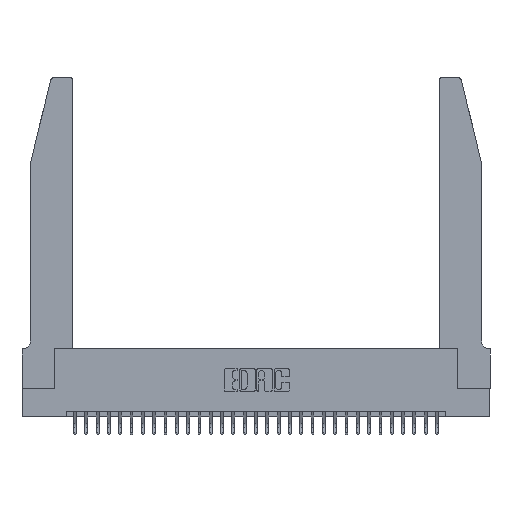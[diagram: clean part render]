
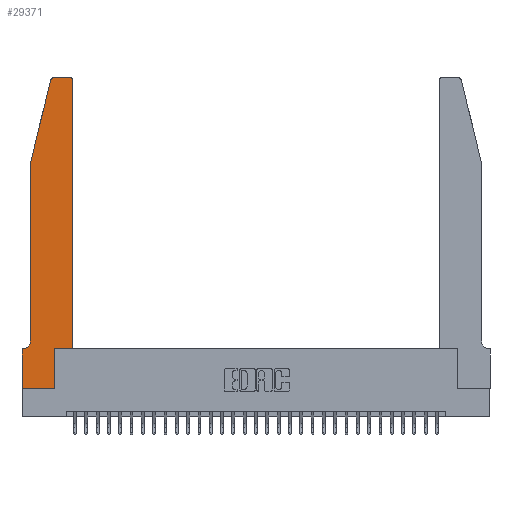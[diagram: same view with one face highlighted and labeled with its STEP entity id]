
A CAD part, top view. The second image highlights one B-rep face of the part: STEP entity #29371.
In plain terms, the highlighted planar face has unit normal (0, 0, 1).
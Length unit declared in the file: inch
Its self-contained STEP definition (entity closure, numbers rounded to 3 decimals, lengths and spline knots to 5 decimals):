
#147 = AXIS2_PLACEMENT_3D ( 'NONE', #3339, #28651, #21407 ) ;
#237 = ORIENTED_EDGE ( 'NONE', *, *, #23715, .T. ) ;
#705 = VERTEX_POINT ( 'NONE', #23378 ) ;
#1278 = VERTEX_POINT ( 'NONE', #14502 ) ;
#1462 = EDGE_CURVE ( 'NONE', #21361, #1278, #31575, .T. ) ;
#1588 = DIRECTION ( 'NONE',  ( -1., 0., 0. ) ) ;
#1649 = DIRECTION ( 'NONE',  ( -1., 0., 0. ) ) ;
#1764 = FACE_OUTER_BOUND ( 'NONE', #12556, .T. ) ;
#1934 = EDGE_CURVE ( 'NONE', #3386, #21623, #21065, .T. ) ;
#2164 = ORIENTED_EDGE ( 'NONE', *, *, #7362, .T. ) ;
#2233 = VERTEX_POINT ( 'NONE', #9811 ) ;
#2481 = CARTESIAN_POINT ( 'NONE',  ( 0., 0., 0.37 ) ) ;
#3025 = CIRCLE ( 'NONE', #10329, 0.07 ) ;
#3180 = ORIENTED_EDGE ( 'NONE', *, *, #1462, .T. ) ;
#3339 = CARTESIAN_POINT ( 'NONE',  ( 0.4205, 2.72, 0.37 ) ) ;
#3386 = VERTEX_POINT ( 'NONE', #26646 ) ;
#3661 = DIRECTION ( 'NONE',  ( 0., -1., 0. ) ) ;
#3945 = ORIENTED_EDGE ( 'NONE', *, *, #8197, .T. ) ;
#4258 = CARTESIAN_POINT ( 'NONE',  ( 0.284, 2.72, 0.37 ) ) ;
#4350 = CARTESIAN_POINT ( 'NONE',  ( 0., 0.35, 0.37 ) ) ;
#4453 = LINE ( 'NONE', #6448, #10668 ) ;
#4527 = CARTESIAN_POINT ( 'NONE',  ( 0., 0., 0.37 ) ) ;
#4607 = CARTESIAN_POINT ( 'NONE',  ( 0., 0.35, 0.37 ) ) ;
#4752 = DIRECTION ( 'NONE',  ( 0., -1., 0. ) ) ;
#5049 = AXIS2_PLACEMENT_3D ( 'NONE', #4258, #14022, #14249 ) ;
#5415 = ORIENTED_EDGE ( 'NONE', *, *, #1934, .T. ) ;
#5787 = CIRCLE ( 'NONE', #5049, 0.03 ) ;
#5803 = ORIENTED_EDGE ( 'NONE', *, *, #11107, .T. ) ;
#6448 = CARTESIAN_POINT ( 'NONE',  ( 0.0755, 0.35, 0.37 ) ) ;
#6578 = VERTEX_POINT ( 'NONE', #4350 ) ;
#6748 = DIRECTION ( 'NONE',  ( 1., 0., 0. ) ) ;
#6808 = ORIENTED_EDGE ( 'NONE', *, *, #9315, .T. ) ;
#6871 = DIRECTION ( 'NONE',  ( 0., 1., 0. ) ) ;
#6883 = LINE ( 'NONE', #14380, #18516 ) ;
#6910 = CARTESIAN_POINT ( 'NONE',  ( 0.2605, 2.75, 0.37 ) ) ;
#6927 = ORIENTED_EDGE ( 'NONE', *, *, #23131, .T. ) ;
#7362 = EDGE_CURVE ( 'NONE', #1278, #29435, #21138, .T. ) ;
#8197 = EDGE_CURVE ( 'NONE', #30524, #21361, #5787, .T. ) ;
#8481 = CARTESIAN_POINT ( 'NONE',  ( 0.4205, 2.75, 0.37 ) ) ;
#8822 = EDGE_CURVE ( 'NONE', #11421, #30524, #29008, .T. ) ;
#9034 = CARTESIAN_POINT ( 'NONE',  ( 0.2865, 0.35, 0.37 ) ) ;
#9295 = VECTOR ( 'NONE', #27070, 39.37008 ) ;
#9315 = EDGE_CURVE ( 'NONE', #705, #11421, #12741, .T. ) ;
#9405 = ORIENTED_EDGE ( 'NONE', *, *, #22620, .T. ) ;
#9459 = DIRECTION ( 'NONE',  ( 0., 0., 1. ) ) ;
#9489 = EDGE_CURVE ( 'NONE', #21623, #705, #6883, .T. ) ;
#9811 = CARTESIAN_POINT ( 'NONE',  ( 0.0055, 0.35, 0.37 ) ) ;
#10329 = AXIS2_PLACEMENT_3D ( 'NONE', #23628, #31355, #1649 ) ;
#10386 = ORIENTED_EDGE ( 'NONE', *, *, #28845, .T. ) ;
#10668 = VECTOR ( 'NONE', #1588, 39.37008 ) ;
#10918 = CARTESIAN_POINT ( 'NONE',  ( 0.0755, 2., 0.37 ) ) ;
#11107 = EDGE_CURVE ( 'NONE', #2233, #6578, #4453, .T. ) ;
#11223 = VECTOR ( 'NONE', #14382, 39.37008 ) ;
#11421 = VERTEX_POINT ( 'NONE', #8481 ) ;
#12450 = LINE ( 'NONE', #17221, #9295 ) ;
#12503 = AXIS2_PLACEMENT_3D ( 'NONE', #4607, #9459, #6748 ) ;
#12556 = EDGE_LOOP ( 'NONE', ( #21592, #3945, #3180, #2164, #237, #5803, #10386, #9405, #6927, #5415, #12750, #6808 ) ) ;
#12741 = CIRCLE ( 'NONE', #147, 0.03 ) ;
#12750 = ORIENTED_EDGE ( 'NONE', *, *, #9489, .T. ) ;
#14022 = DIRECTION ( 'NONE',  ( 0., 0., 1. ) ) ;
#14249 = DIRECTION ( 'NONE',  ( 1., 0., 0. ) ) ;
#14373 = PLANE ( 'NONE',  #12503 ) ;
#14380 = CARTESIAN_POINT ( 'NONE',  ( 0.4505, 0.35, 0.37 ) ) ;
#14382 = DIRECTION ( 'NONE',  ( 0., 1., 0. ) ) ;
#14502 = CARTESIAN_POINT ( 'NONE',  ( 0.0755, 2., 0.37 ) ) ;
#14812 = CARTESIAN_POINT ( 'NONE',  ( 0.0755, 0.42, 0.37 ) ) ;
#16044 = VECTOR ( 'NONE', #21302, 39.37008 ) ;
#16528 = VECTOR ( 'NONE', #4752, 39.37008 ) ;
#16774 = CARTESIAN_POINT ( 'NONE',  ( 0.25487, 2.72718, 0.37 ) ) ;
#17221 = CARTESIAN_POINT ( 'NONE',  ( 0., 0., 0.37 ) ) ;
#18432 = VECTOR ( 'NONE', #3661, 39.37008 ) ;
#18516 = VECTOR ( 'NONE', #6871, 39.37008 ) ;
#18690 = CARTESIAN_POINT ( 'NONE',  ( 0.0755, 2., 0.37 ) ) ;
#19278 = DIRECTION ( 'NONE',  ( -1., 0., 0. ) ) ;
#20878 = CARTESIAN_POINT ( 'NONE',  ( 0.4505, 0.35, 0.37 ) ) ;
#21065 = LINE ( 'NONE', #30001, #27248 ) ;
#21138 = LINE ( 'NONE', #10918, #18432 ) ;
#21302 = DIRECTION ( 'NONE',  ( -0.239, -0.971, 0. ) ) ;
#21361 = VERTEX_POINT ( 'NONE', #16774 ) ;
#21407 = DIRECTION ( 'NONE',  ( 1., 0., 0. ) ) ;
#21592 = ORIENTED_EDGE ( 'NONE', *, *, #8822, .T. ) ;
#21623 = VERTEX_POINT ( 'NONE', #20878 ) ;
#22618 = VERTEX_POINT ( 'NONE', #29554 ) ;
#22620 = EDGE_CURVE ( 'NONE', #25849, #22618, #12450, .T. ) ;
#23131 = EDGE_CURVE ( 'NONE', #22618, #3386, #28661, .T. ) ;
#23378 = CARTESIAN_POINT ( 'NONE',  ( 0.4505, 2.72, 0.37 ) ) ;
#23628 = CARTESIAN_POINT ( 'NONE',  ( 0.0055, 0.42, 0.37 ) ) ;
#23715 = EDGE_CURVE ( 'NONE', #29435, #2233, #3025, .T. ) ;
#25849 = VERTEX_POINT ( 'NONE', #4527 ) ;
#26646 = CARTESIAN_POINT ( 'NONE',  ( 0.2865, 0.35, 0.37 ) ) ;
#27070 = DIRECTION ( 'NONE',  ( 1., 0., 0. ) ) ;
#27248 = VECTOR ( 'NONE', #29682, 39.37008 ) ;
#27408 = LINE ( 'NONE', #2481, #16528 ) ;
#28241 = VECTOR ( 'NONE', #19278, 39.37008 ) ;
#28651 = DIRECTION ( 'NONE',  ( 0., 0., 1. ) ) ;
#28661 = LINE ( 'NONE', #9034, #11223 ) ;
#28845 = EDGE_CURVE ( 'NONE', #6578, #25849, #27408, .T. ) ;
#29008 = LINE ( 'NONE', #6910, #28241 ) ;
#29103 = CARTESIAN_POINT ( 'NONE',  ( 0.284, 2.75, 0.37 ) ) ;
#29371 = ADVANCED_FACE ( 'NONE', ( #1764 ), #14373, .T. ) ;
#29435 = VERTEX_POINT ( 'NONE', #14812 ) ;
#29554 = CARTESIAN_POINT ( 'NONE',  ( 0.2865, 0., 0.37 ) ) ;
#29682 = DIRECTION ( 'NONE',  ( 1., 0., 0. ) ) ;
#30001 = CARTESIAN_POINT ( 'NONE',  ( 0.4505, 0.35, 0.37 ) ) ;
#30524 = VERTEX_POINT ( 'NONE', #29103 ) ;
#31355 = DIRECTION ( 'NONE',  ( 0., 0., -1. ) ) ;
#31575 = LINE ( 'NONE', #18690, #16044 ) ;
